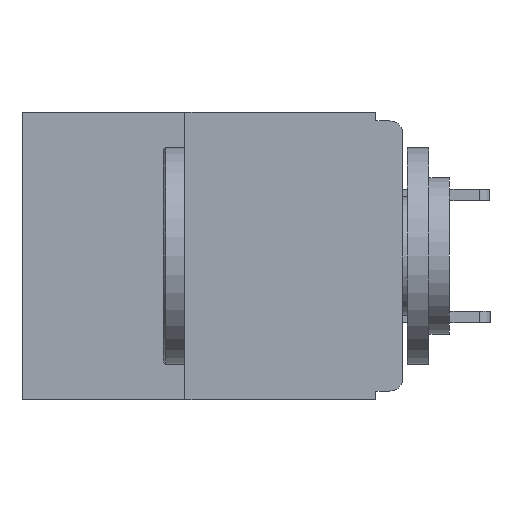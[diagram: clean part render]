
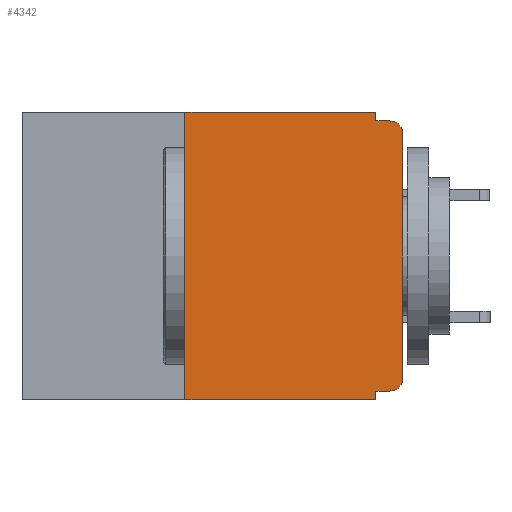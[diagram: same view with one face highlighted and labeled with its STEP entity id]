
A CAD part, left-side view. The second image highlights one B-rep face of the part: STEP entity #4342.
In plain terms, the highlighted planar face has unit normal (-1, 0, 0).
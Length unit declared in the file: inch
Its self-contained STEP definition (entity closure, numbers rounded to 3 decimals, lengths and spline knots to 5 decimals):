
#226 = EDGE_CURVE ( 'NONE', #9652, #14001, #4973, .T. ) ;
#884 = VERTEX_POINT ( 'NONE', #3622 ) ;
#1324 = CARTESIAN_POINT ( 'NONE',  ( 0., 0.031, 0. ) ) ;
#1468 = CARTESIAN_POINT ( 'NONE',  ( 0., 0.031, 0. ) ) ;
#2041 = DIRECTION ( 'NONE',  ( 0., 0., -1. ) ) ;
#2261 = LINE ( 'NONE', #13636, #12084 ) ;
#2545 = VERTEX_POINT ( 'NONE', #10838 ) ;
#2631 = DIRECTION ( 'NONE',  ( 0., -1., 0. ) ) ;
#2669 = DIRECTION ( 'NONE',  ( 1., 0., 0. ) ) ;
#3496 = VECTOR ( 'NONE', #2631, 39.37008 ) ;
#3622 = CARTESIAN_POINT ( 'NONE',  ( 0., 0., -0.025 ) ) ;
#3753 = VERTEX_POINT ( 'NONE', #1468 ) ;
#4342 = ADVANCED_FACE ( 'NONE', ( #23719 ), #24645, .F. ) ;
#4973 = LINE ( 'NONE', #16844, #9634 ) ;
#5275 = VECTOR ( 'NONE', #20364, 39.37008 ) ;
#6369 = ORIENTED_EDGE ( 'NONE', *, *, #226, .F. ) ;
#6507 = CARTESIAN_POINT ( 'NONE',  ( 0., 0.437, 0. ) ) ;
#6797 = CARTESIAN_POINT ( 'NONE',  ( 0., 0.015, -0.025 ) ) ;
#6939 = EDGE_CURVE ( 'NONE', #14931, #884, #2261, .T. ) ;
#7324 = ORIENTED_EDGE ( 'NONE', *, *, #15183, .F. ) ;
#7412 = EDGE_CURVE ( 'NONE', #17226, #14931, #16527, .T. ) ;
#7597 = DIRECTION ( 'NONE',  ( 0., 1., 0. ) ) ;
#7626 = ORIENTED_EDGE ( 'NONE', *, *, #19555, .F. ) ;
#8007 = AXIS2_PLACEMENT_3D ( 'NONE', #6797, #20164, #8808 ) ;
#8808 = DIRECTION ( 'NONE',  ( 0., 0., -1. ) ) ;
#8877 = AXIS2_PLACEMENT_3D ( 'NONE', #22197, #2669, #2041 ) ;
#8891 = ORIENTED_EDGE ( 'NONE', *, *, #18307, .F. ) ;
#9008 = EDGE_LOOP ( 'NONE', ( #11264, #12495, #6369, #7626, #23402, #8891, #15178, #20159, #7324, #12513 ) ) ;
#9304 = DIRECTION ( 'NONE',  ( 0., 0., -1. ) ) ;
#9481 = DIRECTION ( 'NONE',  ( 0., 0., -1. ) ) ;
#9486 = VECTOR ( 'NONE', #9481, 39.37008 ) ;
#9567 = CARTESIAN_POINT ( 'NONE',  ( 0., 0.015, -0.32 ) ) ;
#9634 = VECTOR ( 'NONE', #16769, 39.37008 ) ;
#9652 = VERTEX_POINT ( 'NONE', #13059 ) ;
#10008 = LINE ( 'NONE', #16725, #24475 ) ;
#10171 = VERTEX_POINT ( 'NONE', #20530 ) ;
#10802 = VECTOR ( 'NONE', #9304, 39.37008 ) ;
#10838 = CARTESIAN_POINT ( 'NONE',  ( 0., 0.031, -0.32 ) ) ;
#10866 = AXIS2_PLACEMENT_3D ( 'NONE', #14804, #14799, #14718 ) ;
#11264 = ORIENTED_EDGE ( 'NONE', *, *, #6939, .T. ) ;
#11328 = EDGE_CURVE ( 'NONE', #884, #14001, #18026, .T. ) ;
#11392 = CARTESIAN_POINT ( 'NONE',  ( 0., 0.25, -0.33 ) ) ;
#12084 = VECTOR ( 'NONE', #14387, 39.37008 ) ;
#12495 = ORIENTED_EDGE ( 'NONE', *, *, #11328, .T. ) ;
#12513 = ORIENTED_EDGE ( 'NONE', *, *, #7412, .T. ) ;
#12640 = CARTESIAN_POINT ( 'NONE',  ( 0., 0., -0.305 ) ) ;
#13059 = CARTESIAN_POINT ( 'NONE',  ( 0., 0.031, -0.01 ) ) ;
#13636 = CARTESIAN_POINT ( 'NONE',  ( 0., 0., 0. ) ) ;
#14001 = VERTEX_POINT ( 'NONE', #15243 ) ;
#14009 = VERTEX_POINT ( 'NONE', #11392 ) ;
#14387 = DIRECTION ( 'NONE',  ( 0., 0., 1. ) ) ;
#14584 = LINE ( 'NONE', #18931, #9486 ) ;
#14718 = DIRECTION ( 'NONE',  ( 0., 0., -1. ) ) ;
#14799 = DIRECTION ( 'NONE',  ( -1., 0., 0. ) ) ;
#14804 = CARTESIAN_POINT ( 'NONE',  ( 0., 0.015, -0.305 ) ) ;
#14931 = VERTEX_POINT ( 'NONE', #12640 ) ;
#15178 = ORIENTED_EDGE ( 'NONE', *, *, #17051, .T. ) ;
#15183 = EDGE_CURVE ( 'NONE', #17226, #2545, #18733, .T. ) ;
#15243 = CARTESIAN_POINT ( 'NONE',  ( 0., 0.015, -0.01 ) ) ;
#15803 = EDGE_CURVE ( 'NONE', #2545, #19827, #14584, .T. ) ;
#15881 = CARTESIAN_POINT ( 'NONE',  ( 0., 0.031, -0.33 ) ) ;
#16527 = CIRCLE ( 'NONE', #10866, 0.015 ) ;
#16725 = CARTESIAN_POINT ( 'NONE',  ( 0., 0.437, -0.33 ) ) ;
#16769 = DIRECTION ( 'NONE',  ( 0., -1., 0. ) ) ;
#16844 = CARTESIAN_POINT ( 'NONE',  ( 0., 0., -0.01 ) ) ;
#17051 = EDGE_CURVE ( 'NONE', #14009, #19827, #10008, .T. ) ;
#17226 = VERTEX_POINT ( 'NONE', #9567 ) ;
#18026 = CIRCLE ( 'NONE', #8007, 0.015 ) ;
#18307 = EDGE_CURVE ( 'NONE', #14009, #10171, #20607, .T. ) ;
#18480 = CARTESIAN_POINT ( 'NONE',  ( 0., 0.25, -0.33 ) ) ;
#18621 = DIRECTION ( 'NONE',  ( 0., -1., 0. ) ) ;
#18733 = LINE ( 'NONE', #22824, #23720 ) ;
#18931 = CARTESIAN_POINT ( 'NONE',  ( 0., 0.031, -0.33 ) ) ;
#19555 = EDGE_CURVE ( 'NONE', #3753, #9652, #20874, .T. ) ;
#19827 = VERTEX_POINT ( 'NONE', #15881 ) ;
#20159 = ORIENTED_EDGE ( 'NONE', *, *, #15803, .F. ) ;
#20164 = DIRECTION ( 'NONE',  ( -1., 0., 0. ) ) ;
#20364 = DIRECTION ( 'NONE',  ( 0., 0., 1. ) ) ;
#20530 = CARTESIAN_POINT ( 'NONE',  ( 0., 0.25, 0. ) ) ;
#20607 = LINE ( 'NONE', #18480, #5275 ) ;
#20874 = LINE ( 'NONE', #1324, #10802 ) ;
#22197 = CARTESIAN_POINT ( 'NONE',  ( 0., 0.437, 0. ) ) ;
#22824 = CARTESIAN_POINT ( 'NONE',  ( 0., 0., -0.32 ) ) ;
#23325 = LINE ( 'NONE', #6507, #3496 ) ;
#23351 = EDGE_CURVE ( 'NONE', #10171, #3753, #23325, .T. ) ;
#23402 = ORIENTED_EDGE ( 'NONE', *, *, #23351, .F. ) ;
#23719 = FACE_OUTER_BOUND ( 'NONE', #9008, .T. ) ;
#23720 = VECTOR ( 'NONE', #7597, 39.37008 ) ;
#24475 = VECTOR ( 'NONE', #18621, 39.37008 ) ;
#24645 = PLANE ( 'NONE',  #8877 ) ;
